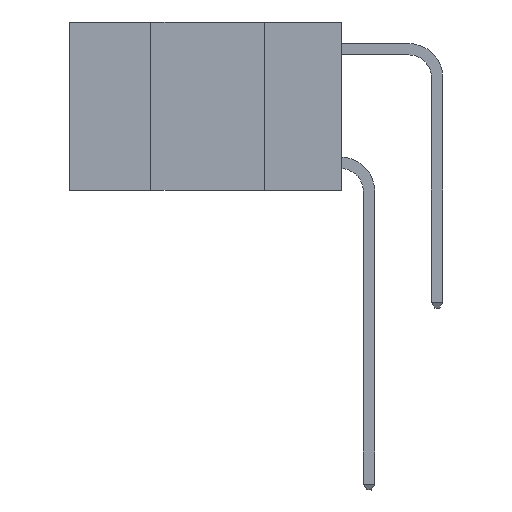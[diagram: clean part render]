
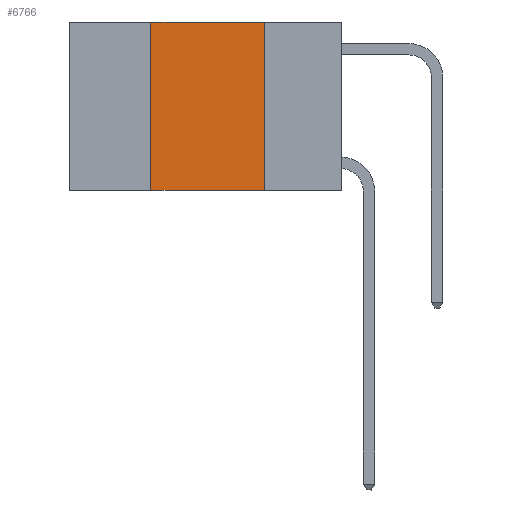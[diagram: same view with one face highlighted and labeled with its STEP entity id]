
A CAD part, left-side view. The second image highlights one B-rep face of the part: STEP entity #6766.
In plain terms, the highlighted planar face has unit normal (-1, 0, 0).
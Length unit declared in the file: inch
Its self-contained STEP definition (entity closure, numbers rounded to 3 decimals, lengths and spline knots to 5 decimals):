
#1427 = CARTESIAN_POINT ( 'NONE',  ( 0., 0.6, -0.37 ) ) ;
#1844 = EDGE_CURVE ( 'NONE', #32032, #5958, #19850, .T. ) ;
#2226 = CARTESIAN_POINT ( 'NONE',  ( 0., 0.17, 0. ) ) ;
#2865 = FACE_OUTER_BOUND ( 'NONE', #21404, .T. ) ;
#3905 = ORIENTED_EDGE ( 'NONE', *, *, #24738, .F. ) ;
#4546 = DIRECTION ( 'NONE',  ( 1., 0., 0. ) ) ;
#5958 = VERTEX_POINT ( 'NONE', #9238 ) ;
#6037 = VECTOR ( 'NONE', #24739, 39.37008 ) ;
#6710 = VECTOR ( 'NONE', #33411, 39.37008 ) ;
#6766 = ADVANCED_FACE ( 'NONE', ( #2865 ), #20077, .F. ) ;
#8398 = AXIS2_PLACEMENT_3D ( 'NONE', #9647, #4546, #22713 ) ;
#9238 = CARTESIAN_POINT ( 'NONE',  ( 0., 0.17, -0.37 ) ) ;
#9647 = CARTESIAN_POINT ( 'NONE',  ( 0., 0.6, 0. ) ) ;
#11095 = ORIENTED_EDGE ( 'NONE', *, *, #1844, .T. ) ;
#11527 = ORIENTED_EDGE ( 'NONE', *, *, #20569, .F. ) ;
#13638 = VECTOR ( 'NONE', #23027, 39.37008 ) ;
#15192 = VERTEX_POINT ( 'NONE', #30189 ) ;
#15255 = LINE ( 'NONE', #2226, #13638 ) ;
#16659 = CARTESIAN_POINT ( 'NONE',  ( 0., 0.42, 0. ) ) ;
#18188 = VECTOR ( 'NONE', #21879, 39.37008 ) ;
#19850 = LINE ( 'NONE', #1427, #6037 ) ;
#20077 = PLANE ( 'NONE',  #8398 ) ;
#20510 = LINE ( 'NONE', #25621, #6710 ) ;
#20569 = EDGE_CURVE ( 'NONE', #15192, #5958, #15255, .T. ) ;
#20599 = EDGE_CURVE ( 'NONE', #32128, #15192, #20510, .T. ) ;
#21404 = EDGE_LOOP ( 'NONE', ( #11527, #22900, #3905, #11095 ) ) ;
#21879 = DIRECTION ( 'NONE',  ( 0., 0., 1. ) ) ;
#22713 = DIRECTION ( 'NONE',  ( 0., 0., -1. ) ) ;
#22900 = ORIENTED_EDGE ( 'NONE', *, *, #20599, .F. ) ;
#23027 = DIRECTION ( 'NONE',  ( 0., 0., -1. ) ) ;
#24738 = EDGE_CURVE ( 'NONE', #32032, #32128, #32768, .T. ) ;
#24739 = DIRECTION ( 'NONE',  ( 0., -1., 0. ) ) ;
#25621 = CARTESIAN_POINT ( 'NONE',  ( 0., 0.6, 0. ) ) ;
#30189 = CARTESIAN_POINT ( 'NONE',  ( 0., 0.17, 0. ) ) ;
#31201 = CARTESIAN_POINT ( 'NONE',  ( 0., 0.42, 0. ) ) ;
#32032 = VERTEX_POINT ( 'NONE', #33464 ) ;
#32128 = VERTEX_POINT ( 'NONE', #31201 ) ;
#32768 = LINE ( 'NONE', #16659, #18188 ) ;
#33411 = DIRECTION ( 'NONE',  ( 0., -1., 0. ) ) ;
#33464 = CARTESIAN_POINT ( 'NONE',  ( 0., 0.42, -0.37 ) ) ;
